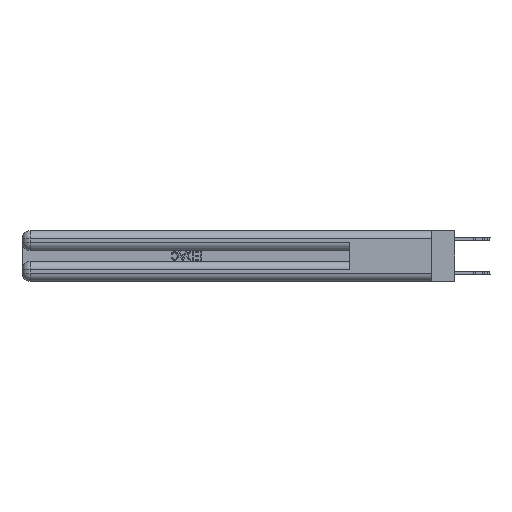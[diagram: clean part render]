
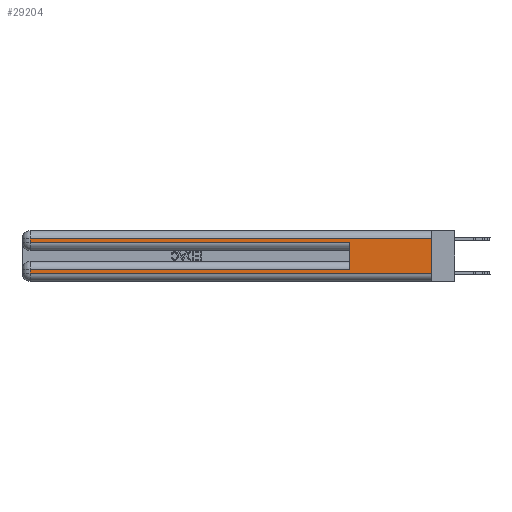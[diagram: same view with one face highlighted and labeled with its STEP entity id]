
A CAD part, left-side view. The second image highlights one B-rep face of the part: STEP entity #29204.
In plain terms, the highlighted planar face has unit normal (-1, 0, 0).
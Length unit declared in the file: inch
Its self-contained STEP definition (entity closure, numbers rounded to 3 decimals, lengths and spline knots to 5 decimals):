
#432 = DIRECTION ( 'NONE',  ( 0., -1., 0. ) ) ;
#685 = VECTOR ( 'NONE', #16663, 39.37008 ) ;
#751 = LINE ( 'NONE', #23298, #10903 ) ;
#1309 = LINE ( 'NONE', #3903, #2471 ) ;
#1571 = CARTESIAN_POINT ( 'NONE',  ( 0., 0., 0.31 ) ) ;
#1588 = CARTESIAN_POINT ( 'NONE',  ( 0., 2.94, 0.085 ) ) ;
#1591 = CARTESIAN_POINT ( 'NONE',  ( 0., 2.94, 0.06 ) ) ;
#2232 = CARTESIAN_POINT ( 'NONE',  ( 0., 0., 0.285 ) ) ;
#2280 = CARTESIAN_POINT ( 'NONE',  ( 0., 0., 0.085 ) ) ;
#2471 = VECTOR ( 'NONE', #13779, 39.37008 ) ;
#3812 = ORIENTED_EDGE ( 'NONE', *, *, #31821, .T. ) ;
#3903 = CARTESIAN_POINT ( 'NONE',  ( 0., 2.94, 0.37 ) ) ;
#4150 = VECTOR ( 'NONE', #22402, 39.37008 ) ;
#4765 = VERTEX_POINT ( 'NONE', #9275 ) ;
#5418 = DIRECTION ( 'NONE',  ( 1., 0., 0. ) ) ;
#5430 = VECTOR ( 'NONE', #15199, 39.37008 ) ;
#5674 = EDGE_CURVE ( 'NONE', #16496, #19079, #751, .T. ) ;
#6684 = CARTESIAN_POINT ( 'NONE',  ( 0., 0., 0.06 ) ) ;
#6746 = ORIENTED_EDGE ( 'NONE', *, *, #14085, .T. ) ;
#7015 = ORIENTED_EDGE ( 'NONE', *, *, #30311, .T. ) ;
#7366 = PLANE ( 'NONE',  #31301 ) ;
#7469 = LINE ( 'NONE', #2280, #17199 ) ;
#7685 = FACE_OUTER_BOUND ( 'NONE', #19658, .T. ) ;
#7714 = LINE ( 'NONE', #17455, #20790 ) ;
#9275 = CARTESIAN_POINT ( 'NONE',  ( 0., 2.94, 0.31 ) ) ;
#10056 = DIRECTION ( 'NONE',  ( 0., 1., 0. ) ) ;
#10130 = VERTEX_POINT ( 'NONE', #31258 ) ;
#10340 = VERTEX_POINT ( 'NONE', #13043 ) ;
#10903 = VECTOR ( 'NONE', #432, 39.37008 ) ;
#11302 = LINE ( 'NONE', #1571, #685 ) ;
#12324 = LINE ( 'NONE', #14919, #4150 ) ;
#13043 = CARTESIAN_POINT ( 'NONE',  ( 0., 2.94, 0.285 ) ) ;
#13411 = CARTESIAN_POINT ( 'NONE',  ( 0., 0., 0.31 ) ) ;
#13779 = DIRECTION ( 'NONE',  ( 0., 0., -1. ) ) ;
#14085 = EDGE_CURVE ( 'NONE', #21231, #16496, #1309, .T. ) ;
#14919 = CARTESIAN_POINT ( 'NONE',  ( 0., 2.94, 0.37 ) ) ;
#15030 = LINE ( 'NONE', #2232, #5430 ) ;
#15199 = DIRECTION ( 'NONE',  ( 0., -1., 0. ) ) ;
#15992 = DIRECTION ( 'NONE',  ( 0., 0., 1. ) ) ;
#16496 = VERTEX_POINT ( 'NONE', #1591 ) ;
#16663 = DIRECTION ( 'NONE',  ( 0., 1., 0. ) ) ;
#17199 = VECTOR ( 'NONE', #10056, 39.37008 ) ;
#17455 = CARTESIAN_POINT ( 'NONE',  ( 0., 0., 0.37 ) ) ;
#17952 = DIRECTION ( 'NONE',  ( 0., 0., -1. ) ) ;
#19079 = VERTEX_POINT ( 'NONE', #6684 ) ;
#19658 = EDGE_LOOP ( 'NONE', ( #27066, #7015, #22041, #3812, #26104, #23352, #6746, #29902 ) ) ;
#19773 = EDGE_CURVE ( 'NONE', #26452, #19079, #7714, .T. ) ;
#20339 = EDGE_CURVE ( 'NONE', #22739, #10130, #25602, .T. ) ;
#20790 = VECTOR ( 'NONE', #17952, 39.37008 ) ;
#20969 = EDGE_CURVE ( 'NONE', #4765, #10340, #12324, .T. ) ;
#21231 = VERTEX_POINT ( 'NONE', #1588 ) ;
#22041 = ORIENTED_EDGE ( 'NONE', *, *, #20969, .T. ) ;
#22402 = DIRECTION ( 'NONE',  ( 0., 0., -1. ) ) ;
#22730 = CARTESIAN_POINT ( 'NONE',  ( 0., 0.6, 0.085 ) ) ;
#22739 = VERTEX_POINT ( 'NONE', #22730 ) ;
#22813 = EDGE_CURVE ( 'NONE', #22739, #21231, #7469, .T. ) ;
#23298 = CARTESIAN_POINT ( 'NONE',  ( 0., 0., 0.06 ) ) ;
#23352 = ORIENTED_EDGE ( 'NONE', *, *, #22813, .T. ) ;
#23626 = CARTESIAN_POINT ( 'NONE',  ( 0., 0.6, 0.145 ) ) ;
#25602 = LINE ( 'NONE', #23626, #31102 ) ;
#26104 = ORIENTED_EDGE ( 'NONE', *, *, #20339, .F. ) ;
#26452 = VERTEX_POINT ( 'NONE', #13411 ) ;
#27066 = ORIENTED_EDGE ( 'NONE', *, *, #19773, .F. ) ;
#29204 = ADVANCED_FACE ( 'NONE', ( #7685 ), #7366, .F. ) ;
#29779 = CARTESIAN_POINT ( 'NONE',  ( 0., 0., 0.37 ) ) ;
#29902 = ORIENTED_EDGE ( 'NONE', *, *, #5674, .T. ) ;
#29940 = DIRECTION ( 'NONE',  ( 0., 0., -1. ) ) ;
#30311 = EDGE_CURVE ( 'NONE', #26452, #4765, #11302, .T. ) ;
#31102 = VECTOR ( 'NONE', #15992, 39.37008 ) ;
#31258 = CARTESIAN_POINT ( 'NONE',  ( 0., 0.6, 0.285 ) ) ;
#31301 = AXIS2_PLACEMENT_3D ( 'NONE', #29779, #5418, #29940 ) ;
#31821 = EDGE_CURVE ( 'NONE', #10340, #10130, #15030, .T. ) ;
